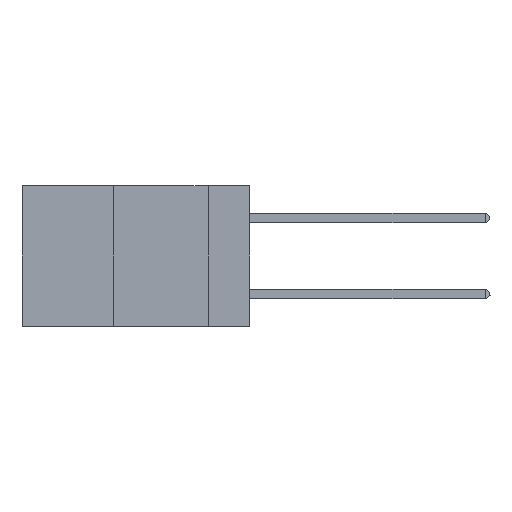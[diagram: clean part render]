
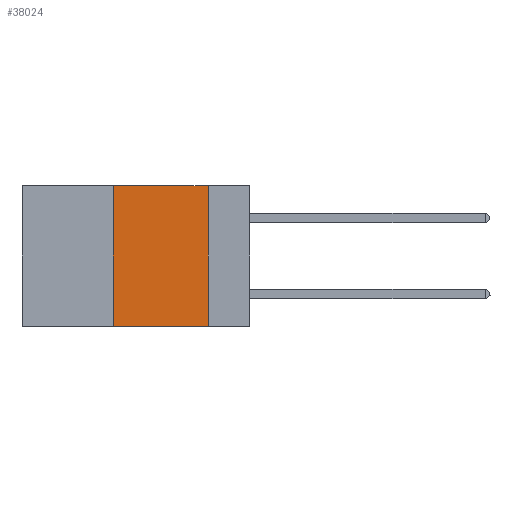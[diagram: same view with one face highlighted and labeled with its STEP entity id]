
A CAD part, left-side view. The second image highlights one B-rep face of the part: STEP entity #38024.
In plain terms, the highlighted planar face has unit normal (-1, 0, 0).
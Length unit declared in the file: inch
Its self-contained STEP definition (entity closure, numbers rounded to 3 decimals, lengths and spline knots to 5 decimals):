
#139 = EDGE_CURVE ( 'NONE', #10131, #36100, #34561, .T. ) ;
#1475 = DIRECTION ( 'NONE',  ( 0., 0., -1. ) ) ;
#1504 = CARTESIAN_POINT ( 'NONE',  ( 0., 0.36, 0. ) ) ;
#2549 = DIRECTION ( 'NONE',  ( 0., -1., 0. ) ) ;
#4358 = CARTESIAN_POINT ( 'NONE',  ( 0., 0.6, 0. ) ) ;
#4816 = DIRECTION ( 'NONE',  ( 1., 0., 0. ) ) ;
#5609 = LINE ( 'NONE', #19822, #27534 ) ;
#8102 = EDGE_LOOP ( 'NONE', ( #14732, #40444, #41842, #41796 ) ) ;
#10131 = VERTEX_POINT ( 'NONE', #41443 ) ;
#13013 = EDGE_CURVE ( 'NONE', #27930, #10131, #14505, .T. ) ;
#14505 = LINE ( 'NONE', #1504, #37911 ) ;
#14732 = ORIENTED_EDGE ( 'NONE', *, *, #18365, .F. ) ;
#15860 = DIRECTION ( 'NONE',  ( 0., 0., -1. ) ) ;
#18365 = EDGE_CURVE ( 'NONE', #36100, #19364, #5609, .T. ) ;
#18722 = VECTOR ( 'NONE', #33616, 39.37008 ) ;
#19364 = VERTEX_POINT ( 'NONE', #26736 ) ;
#19748 = FACE_OUTER_BOUND ( 'NONE', #8102, .T. ) ;
#19822 = CARTESIAN_POINT ( 'NONE',  ( 0., 0.11, 0. ) ) ;
#20970 = DIRECTION ( 'NONE',  ( 0., 0., 1. ) ) ;
#22389 = VECTOR ( 'NONE', #2549, 39.37008 ) ;
#24217 = CARTESIAN_POINT ( 'NONE',  ( 0., 0.6, 0. ) ) ;
#26736 = CARTESIAN_POINT ( 'NONE',  ( 0., 0.11, -0.37 ) ) ;
#27534 = VECTOR ( 'NONE', #15860, 39.37008 ) ;
#27930 = VERTEX_POINT ( 'NONE', #35130 ) ;
#28440 = EDGE_CURVE ( 'NONE', #27930, #19364, #31038, .T. ) ;
#29306 = CARTESIAN_POINT ( 'NONE',  ( 0., 0.11, 0. ) ) ;
#31038 = LINE ( 'NONE', #31736, #22389 ) ;
#31736 = CARTESIAN_POINT ( 'NONE',  ( 0., 0.6, -0.37 ) ) ;
#33616 = DIRECTION ( 'NONE',  ( 0., -1., 0. ) ) ;
#33661 = PLANE ( 'NONE',  #35083 ) ;
#34561 = LINE ( 'NONE', #4358, #18722 ) ;
#35083 = AXIS2_PLACEMENT_3D ( 'NONE', #24217, #4816, #1475 ) ;
#35130 = CARTESIAN_POINT ( 'NONE',  ( 0., 0.36, -0.37 ) ) ;
#36100 = VERTEX_POINT ( 'NONE', #29306 ) ;
#37911 = VECTOR ( 'NONE', #20970, 39.37008 ) ;
#38024 = ADVANCED_FACE ( 'NONE', ( #19748 ), #33661, .F. ) ;
#40444 = ORIENTED_EDGE ( 'NONE', *, *, #139, .F. ) ;
#41443 = CARTESIAN_POINT ( 'NONE',  ( 0., 0.36, 0. ) ) ;
#41796 = ORIENTED_EDGE ( 'NONE', *, *, #28440, .T. ) ;
#41842 = ORIENTED_EDGE ( 'NONE', *, *, #13013, .F. ) ;
